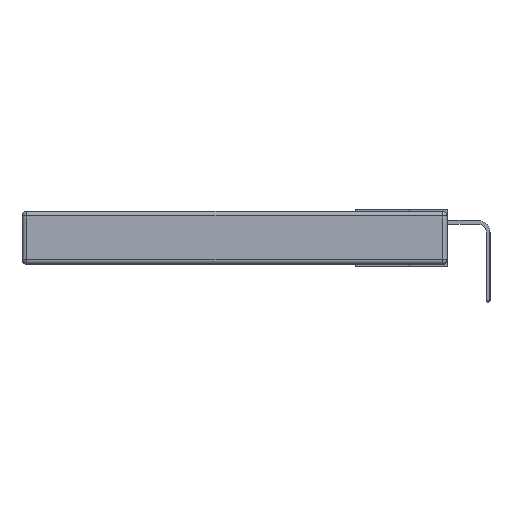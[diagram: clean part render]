
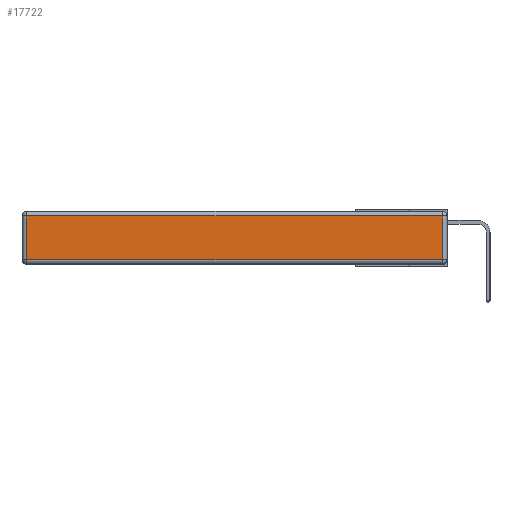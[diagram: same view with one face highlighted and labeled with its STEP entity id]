
A CAD part, left-side view. The second image highlights one B-rep face of the part: STEP entity #17722.
In plain terms, the highlighted planar face has unit normal (-1, 0, 0).
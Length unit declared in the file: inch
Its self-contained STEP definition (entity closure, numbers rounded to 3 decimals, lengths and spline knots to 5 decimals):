
#32 = CARTESIAN_POINT ( 'NONE',  ( 0., 2.75, -0.03 ) ) ;
#339 = EDGE_CURVE ( 'NONE', #13407, #2077, #1463, .T. ) ;
#807 = CARTESIAN_POINT ( 'NONE',  ( 0., 0.03, -0.343 ) ) ;
#1463 = LINE ( 'NONE', #32, #4179 ) ;
#1840 = EDGE_CURVE ( 'NONE', #10526, #13407, #17895, .T. ) ;
#1900 = DIRECTION ( 'NONE',  ( 0., 0., 1. ) ) ;
#1974 = PLANE ( 'NONE',  #23765 ) ;
#2077 = VERTEX_POINT ( 'NONE', #20832 ) ;
#2329 = LINE ( 'NONE', #5883, #6842 ) ;
#3686 = VECTOR ( 'NONE', #5327, 39.37008 ) ;
#4179 = VECTOR ( 'NONE', #7666, 39.37008 ) ;
#4315 = ORIENTED_EDGE ( 'NONE', *, *, #4834, .T. ) ;
#4834 = EDGE_CURVE ( 'NONE', #2077, #10502, #24082, .T. ) ;
#5327 = DIRECTION ( 'NONE',  ( 0., 0., -1. ) ) ;
#5883 = CARTESIAN_POINT ( 'NONE',  ( 0., 0., -0.313 ) ) ;
#6842 = VECTOR ( 'NONE', #13843, 39.37008 ) ;
#7064 = FACE_OUTER_BOUND ( 'NONE', #24431, .T. ) ;
#7666 = DIRECTION ( 'NONE',  ( 0., 1., 0. ) ) ;
#10502 = VERTEX_POINT ( 'NONE', #13963 ) ;
#10526 = VERTEX_POINT ( 'NONE', #13485 ) ;
#10985 = ORIENTED_EDGE ( 'NONE', *, *, #1840, .T. ) ;
#11407 = CARTESIAN_POINT ( 'NONE',  ( 0., 0., -0.343 ) ) ;
#11911 = VECTOR ( 'NONE', #20073, 39.37008 ) ;
#13407 = VERTEX_POINT ( 'NONE', #16338 ) ;
#13443 = DIRECTION ( 'NONE',  ( -1., 0., 0. ) ) ;
#13485 = CARTESIAN_POINT ( 'NONE',  ( 0., 0.03, -0.313 ) ) ;
#13843 = DIRECTION ( 'NONE',  ( 0., -1., 0. ) ) ;
#13963 = CARTESIAN_POINT ( 'NONE',  ( 0., 2.72, -0.313 ) ) ;
#14484 = EDGE_CURVE ( 'NONE', #10502, #10526, #2329, .T. ) ;
#16338 = CARTESIAN_POINT ( 'NONE',  ( 0., 0.03, -0.03 ) ) ;
#16578 = CARTESIAN_POINT ( 'NONE',  ( 0., 2.72, -0.343 ) ) ;
#17722 = ADVANCED_FACE ( 'NONE', ( #7064 ), #1974, .T. ) ;
#17779 = ORIENTED_EDGE ( 'NONE', *, *, #14484, .T. ) ;
#17895 = LINE ( 'NONE', #807, #11911 ) ;
#20073 = DIRECTION ( 'NONE',  ( 0., 0., 1. ) ) ;
#20832 = CARTESIAN_POINT ( 'NONE',  ( 0., 2.72, -0.03 ) ) ;
#21901 = ORIENTED_EDGE ( 'NONE', *, *, #339, .T. ) ;
#23765 = AXIS2_PLACEMENT_3D ( 'NONE', #11407, #13443, #1900 ) ;
#24082 = LINE ( 'NONE', #16578, #3686 ) ;
#24431 = EDGE_LOOP ( 'NONE', ( #17779, #10985, #21901, #4315 ) ) ;
